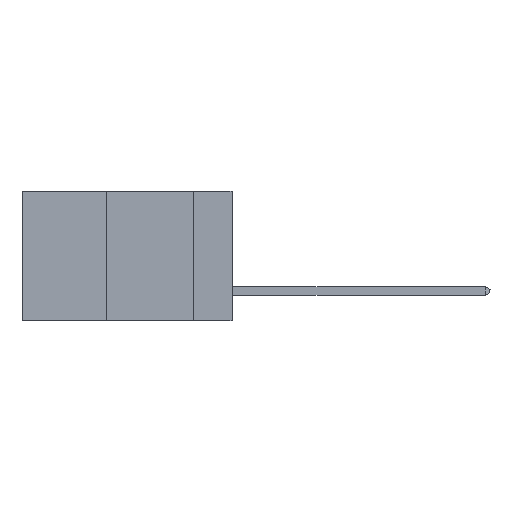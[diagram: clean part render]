
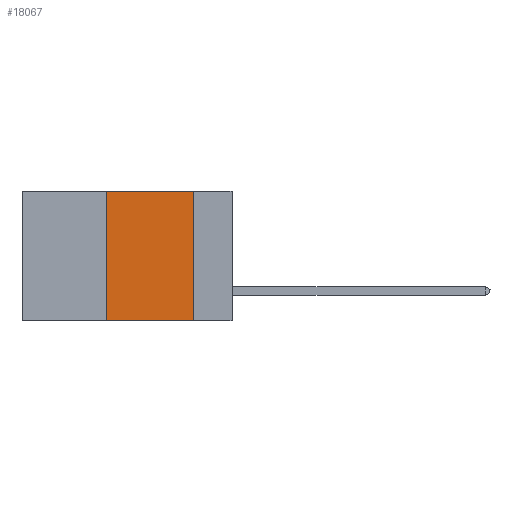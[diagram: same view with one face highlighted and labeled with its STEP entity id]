
A CAD part, left-side view. The second image highlights one B-rep face of the part: STEP entity #18067.
In plain terms, the highlighted planar face has unit normal (-1, 0, 0).
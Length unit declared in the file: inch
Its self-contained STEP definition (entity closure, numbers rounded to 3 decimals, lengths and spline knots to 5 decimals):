
#777 = VECTOR ( 'NONE', #6294, 39.37008 ) ;
#2476 = ORIENTED_EDGE ( 'NONE', *, *, #6093, .F. ) ;
#6093 = EDGE_CURVE ( 'NONE', #7642, #16980, #6299, .T. ) ;
#6294 = DIRECTION ( 'NONE',  ( 0., 0., 1. ) ) ;
#6299 = LINE ( 'NONE', #11199, #14225 ) ;
#6340 = VERTEX_POINT ( 'NONE', #10166 ) ;
#6400 = LINE ( 'NONE', #35337, #13057 ) ;
#7275 = CARTESIAN_POINT ( 'NONE',  ( 0., 0.11, 0. ) ) ;
#7374 = CARTESIAN_POINT ( 'NONE',  ( 0., 0.6, 0. ) ) ;
#7642 = VERTEX_POINT ( 'NONE', #22785 ) ;
#9186 = ORIENTED_EDGE ( 'NONE', *, *, #25735, .T. ) ;
#10166 = CARTESIAN_POINT ( 'NONE',  ( 0., 0.11, -0.37 ) ) ;
#10220 = DIRECTION ( 'NONE',  ( 0., 0., -1. ) ) ;
#10425 = VERTEX_POINT ( 'NONE', #12547 ) ;
#11199 = CARTESIAN_POINT ( 'NONE',  ( 0., 0.6, 0. ) ) ;
#12547 = CARTESIAN_POINT ( 'NONE',  ( 0., 0.36, -0.37 ) ) ;
#13057 = VECTOR ( 'NONE', #19085, 39.37008 ) ;
#13668 = EDGE_LOOP ( 'NONE', ( #24425, #2476, #15764, #9186 ) ) ;
#14225 = VECTOR ( 'NONE', #14773, 39.37008 ) ;
#14762 = VECTOR ( 'NONE', #27743, 39.37008 ) ;
#14773 = DIRECTION ( 'NONE',  ( 0., -1., 0. ) ) ;
#15764 = ORIENTED_EDGE ( 'NONE', *, *, #31578, .F. ) ;
#16980 = VERTEX_POINT ( 'NONE', #7275 ) ;
#18067 = ADVANCED_FACE ( 'NONE', ( #24645 ), #35868, .F. ) ;
#18295 = CARTESIAN_POINT ( 'NONE',  ( 0., 0.6, -0.37 ) ) ;
#19085 = DIRECTION ( 'NONE',  ( 0., 0., -1. ) ) ;
#22785 = CARTESIAN_POINT ( 'NONE',  ( 0., 0.36, 0. ) ) ;
#24175 = DIRECTION ( 'NONE',  ( 1., 0., 0. ) ) ;
#24425 = ORIENTED_EDGE ( 'NONE', *, *, #28557, .F. ) ;
#24645 = FACE_OUTER_BOUND ( 'NONE', #13668, .T. ) ;
#25735 = EDGE_CURVE ( 'NONE', #10425, #6340, #28339, .T. ) ;
#27743 = DIRECTION ( 'NONE',  ( 0., -1., 0. ) ) ;
#28339 = LINE ( 'NONE', #18295, #14762 ) ;
#28557 = EDGE_CURVE ( 'NONE', #16980, #6340, #6400, .T. ) ;
#30111 = LINE ( 'NONE', #31223, #777 ) ;
#31223 = CARTESIAN_POINT ( 'NONE',  ( 0., 0.36, 0. ) ) ;
#31578 = EDGE_CURVE ( 'NONE', #10425, #7642, #30111, .T. ) ;
#34630 = AXIS2_PLACEMENT_3D ( 'NONE', #7374, #24175, #10220 ) ;
#35337 = CARTESIAN_POINT ( 'NONE',  ( 0., 0.11, 0. ) ) ;
#35868 = PLANE ( 'NONE',  #34630 ) ;
